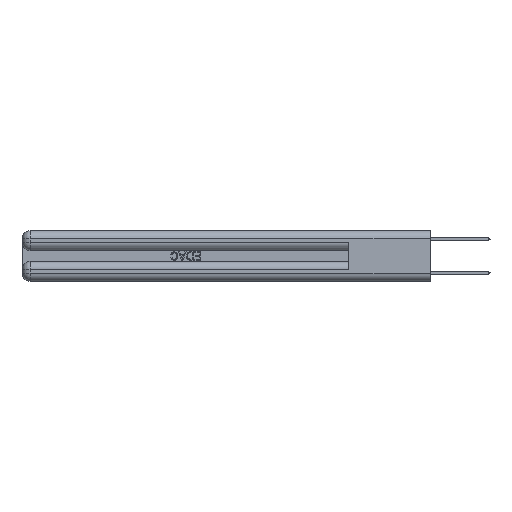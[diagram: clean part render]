
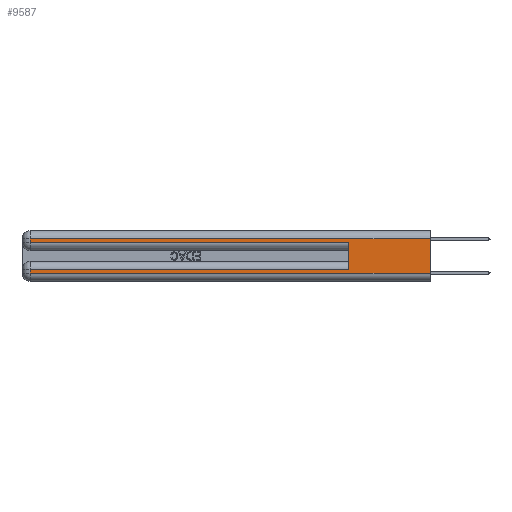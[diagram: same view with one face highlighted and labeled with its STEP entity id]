
A CAD part, left-side view. The second image highlights one B-rep face of the part: STEP entity #9587.
In plain terms, the highlighted planar face has unit normal (-1, 0, 0).
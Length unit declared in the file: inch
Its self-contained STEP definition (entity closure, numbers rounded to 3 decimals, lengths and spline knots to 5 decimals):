
#341 = VECTOR ( 'NONE', #18361, 39.37008 ) ;
#732 = CARTESIAN_POINT ( 'NONE',  ( 0., 0.6, 0.085 ) ) ;
#1258 = CARTESIAN_POINT ( 'NONE',  ( 0., 2.94, 0.37 ) ) ;
#1487 = ORIENTED_EDGE ( 'NONE', *, *, #10011, .T. ) ;
#1537 = EDGE_CURVE ( 'NONE', #22852, #4243, #9003, .T. ) ;
#2330 = PLANE ( 'NONE',  #6197 ) ;
#2358 = ORIENTED_EDGE ( 'NONE', *, *, #1537, .T. ) ;
#2619 = VERTEX_POINT ( 'NONE', #30507 ) ;
#2779 = EDGE_LOOP ( 'NONE', ( #3799, #1487, #28954, #13047, #16665, #2358, #26369, #16849 ) ) ;
#3799 = ORIENTED_EDGE ( 'NONE', *, *, #13526, .F. ) ;
#3927 = LINE ( 'NONE', #1258, #21301 ) ;
#4013 = CARTESIAN_POINT ( 'NONE',  ( 0., 0.6, 0.145 ) ) ;
#4117 = DIRECTION ( 'NONE',  ( 0., 1., 0. ) ) ;
#4157 = DIRECTION ( 'NONE',  ( 0., 0., -1. ) ) ;
#4243 = VERTEX_POINT ( 'NONE', #24285 ) ;
#4292 = LINE ( 'NONE', #7137, #7947 ) ;
#5165 = CARTESIAN_POINT ( 'NONE',  ( 0., 2.94, 0.37 ) ) ;
#6197 = AXIS2_PLACEMENT_3D ( 'NONE', #6999, #22734, #4157 ) ;
#6644 = EDGE_CURVE ( 'NONE', #22852, #6781, #16413, .T. ) ;
#6781 = VERTEX_POINT ( 'NONE', #17745 ) ;
#6999 = CARTESIAN_POINT ( 'NONE',  ( 0., 0., 0.37 ) ) ;
#7137 = CARTESIAN_POINT ( 'NONE',  ( 0., 0., 0.37 ) ) ;
#7319 = VECTOR ( 'NONE', #4117, 39.37008 ) ;
#7518 = LINE ( 'NONE', #5165, #10043 ) ;
#7905 = VERTEX_POINT ( 'NONE', #13945 ) ;
#7947 = VECTOR ( 'NONE', #14494, 39.37008 ) ;
#9003 = LINE ( 'NONE', #16866, #9443 ) ;
#9150 = CARTESIAN_POINT ( 'NONE',  ( 0., 0., 0.31 ) ) ;
#9443 = VECTOR ( 'NONE', #27401, 39.37008 ) ;
#9587 = ADVANCED_FACE ( 'NONE', ( #15027 ), #2330, .F. ) ;
#10011 = EDGE_CURVE ( 'NONE', #29764, #16880, #27546, .T. ) ;
#10043 = VECTOR ( 'NONE', #12690, 39.37008 ) ;
#11523 = EDGE_CURVE ( 'NONE', #4243, #7905, #3927, .T. ) ;
#12690 = DIRECTION ( 'NONE',  ( 0., 0., -1. ) ) ;
#12761 = EDGE_CURVE ( 'NONE', #16880, #2619, #7518, .T. ) ;
#13047 = ORIENTED_EDGE ( 'NONE', *, *, #16022, .T. ) ;
#13415 = VECTOR ( 'NONE', #14381, 39.37008 ) ;
#13526 = EDGE_CURVE ( 'NONE', #29764, #27671, #4292, .T. ) ;
#13945 = CARTESIAN_POINT ( 'NONE',  ( 0., 2.94, 0.06 ) ) ;
#14381 = DIRECTION ( 'NONE',  ( 0., -1., 0. ) ) ;
#14494 = DIRECTION ( 'NONE',  ( 0., 0., -1. ) ) ;
#14540 = LINE ( 'NONE', #19576, #13415 ) ;
#15027 = FACE_OUTER_BOUND ( 'NONE', #2779, .T. ) ;
#16022 = EDGE_CURVE ( 'NONE', #2619, #6781, #14540, .T. ) ;
#16030 = VECTOR ( 'NONE', #29296, 39.37008 ) ;
#16413 = LINE ( 'NONE', #4013, #16030 ) ;
#16665 = ORIENTED_EDGE ( 'NONE', *, *, #6644, .F. ) ;
#16849 = ORIENTED_EDGE ( 'NONE', *, *, #25279, .T. ) ;
#16866 = CARTESIAN_POINT ( 'NONE',  ( 0., 0., 0.085 ) ) ;
#16880 = VERTEX_POINT ( 'NONE', #16950 ) ;
#16950 = CARTESIAN_POINT ( 'NONE',  ( 0., 2.94, 0.31 ) ) ;
#17745 = CARTESIAN_POINT ( 'NONE',  ( 0., 0.6, 0.285 ) ) ;
#18361 = DIRECTION ( 'NONE',  ( 0., -1., 0. ) ) ;
#19576 = CARTESIAN_POINT ( 'NONE',  ( 0., 0., 0.285 ) ) ;
#20526 = CARTESIAN_POINT ( 'NONE',  ( 0., 0., 0.06 ) ) ;
#21186 = DIRECTION ( 'NONE',  ( 0., 0., -1. ) ) ;
#21301 = VECTOR ( 'NONE', #21186, 39.37008 ) ;
#22734 = DIRECTION ( 'NONE',  ( 1., 0., 0. ) ) ;
#22852 = VERTEX_POINT ( 'NONE', #732 ) ;
#23486 = CARTESIAN_POINT ( 'NONE',  ( 0., 0., 0.31 ) ) ;
#24285 = CARTESIAN_POINT ( 'NONE',  ( 0., 2.94, 0.085 ) ) ;
#25279 = EDGE_CURVE ( 'NONE', #7905, #27671, #28054, .T. ) ;
#26369 = ORIENTED_EDGE ( 'NONE', *, *, #11523, .T. ) ;
#27268 = CARTESIAN_POINT ( 'NONE',  ( 0., 0., 0.06 ) ) ;
#27401 = DIRECTION ( 'NONE',  ( 0., 1., 0. ) ) ;
#27546 = LINE ( 'NONE', #9150, #7319 ) ;
#27671 = VERTEX_POINT ( 'NONE', #27268 ) ;
#28054 = LINE ( 'NONE', #20526, #341 ) ;
#28954 = ORIENTED_EDGE ( 'NONE', *, *, #12761, .T. ) ;
#29296 = DIRECTION ( 'NONE',  ( 0., 0., 1. ) ) ;
#29764 = VERTEX_POINT ( 'NONE', #23486 ) ;
#30507 = CARTESIAN_POINT ( 'NONE',  ( 0., 2.94, 0.285 ) ) ;
